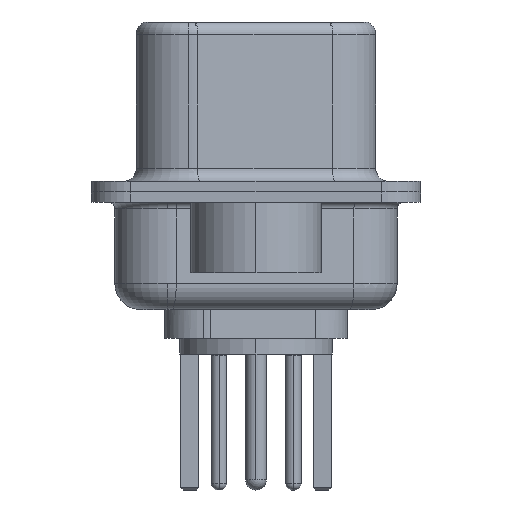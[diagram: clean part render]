
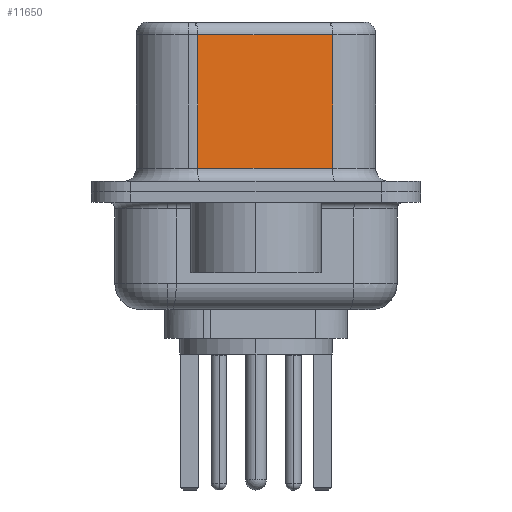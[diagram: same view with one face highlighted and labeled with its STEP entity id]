
A CAD part, left-side view. The second image highlights one B-rep face of the part: STEP entity #11650.
In plain terms, the highlighted planar face has unit normal (-0.985, -0.174, 0).
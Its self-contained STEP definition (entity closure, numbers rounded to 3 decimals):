
#316 = CARTESIAN_POINT ( 'NONE',  ( 4.58, -2.927, 6.02 ) ) ;
#691 = EDGE_CURVE ( 'NONE', #12533, #19667, #10380, .T. ) ;
#2253 = VECTOR ( 'NONE', #14697, 1000. ) ;
#2531 = VECTOR ( 'NONE', #11582, 1000. ) ;
#2867 = LINE ( 'NONE', #22674, #22081 ) ;
#3387 = FACE_OUTER_BOUND ( 'NONE', #6460, .T. ) ;
#4191 = DIRECTION ( 'NONE',  ( 0.174, -0.985, 0. ) ) ;
#5225 = DIRECTION ( 'NONE',  ( -0.174, 0.985, 0. ) ) ;
#6460 = EDGE_LOOP ( 'NONE', ( #8907, #9455, #9629, #20340 ) ) ;
#6999 = PLANE ( 'NONE',  #9494 ) ;
#8251 = CARTESIAN_POINT ( 'NONE',  ( 3.67, 2.233, 0.9 ) ) ;
#8907 = ORIENTED_EDGE ( 'NONE', *, *, #691, .F. ) ;
#9455 = ORIENTED_EDGE ( 'NONE', *, *, #23116, .T. ) ;
#9494 = AXIS2_PLACEMENT_3D ( 'NONE', #18238, #16440, #5225 ) ;
#9497 = EDGE_CURVE ( 'NONE', #14494, #19667, #2867, .T. ) ;
#9629 = ORIENTED_EDGE ( 'NONE', *, *, #22918, .T. ) ;
#10380 = LINE ( 'NONE', #14343, #19705 ) ;
#11582 = DIRECTION ( 'NONE',  ( -0.174, 0.985, 0. ) ) ;
#11650 = ADVANCED_FACE ( 'NONE', ( #3387 ), #6999, .F. ) ;
#12533 = VERTEX_POINT ( 'NONE', #18841 ) ;
#14343 = CARTESIAN_POINT ( 'NONE',  ( 4.58, -2.927, 6.52 ) ) ;
#14494 = VERTEX_POINT ( 'NONE', #8251 ) ;
#14697 = DIRECTION ( 'NONE',  ( 0., 0., -1. ) ) ;
#14890 = CARTESIAN_POINT ( 'NONE',  ( 4.58, -2.927, 0.9 ) ) ;
#16440 = DIRECTION ( 'NONE',  ( 0.985, 0.174, 0. ) ) ;
#16950 = LINE ( 'NONE', #316, #2531 ) ;
#18238 = CARTESIAN_POINT ( 'NONE',  ( 4.58, -2.927, 6.52 ) ) ;
#18463 = VERTEX_POINT ( 'NONE', #23547 ) ;
#18841 = CARTESIAN_POINT ( 'NONE',  ( 4.58, -2.927, 6.02 ) ) ;
#19667 = VERTEX_POINT ( 'NONE', #14890 ) ;
#19705 = VECTOR ( 'NONE', #23364, 1000. ) ;
#20266 = CARTESIAN_POINT ( 'NONE',  ( 3.67, 2.233, 6.52 ) ) ;
#20340 = ORIENTED_EDGE ( 'NONE', *, *, #9497, .T. ) ;
#21516 = LINE ( 'NONE', #20266, #2253 ) ;
#22081 = VECTOR ( 'NONE', #4191, 1000. ) ;
#22674 = CARTESIAN_POINT ( 'NONE',  ( 4.58, -2.927, 0.9 ) ) ;
#22918 = EDGE_CURVE ( 'NONE', #18463, #14494, #21516, .T. ) ;
#23116 = EDGE_CURVE ( 'NONE', #12533, #18463, #16950, .T. ) ;
#23364 = DIRECTION ( 'NONE',  ( 0., 0., -1. ) ) ;
#23547 = CARTESIAN_POINT ( 'NONE',  ( 3.67, 2.233, 6.02 ) ) ;
